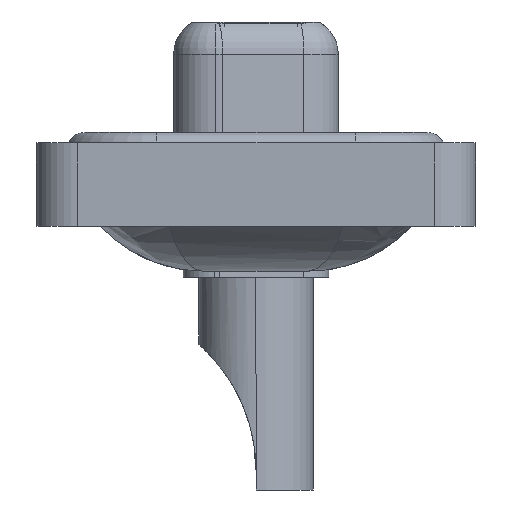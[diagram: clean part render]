
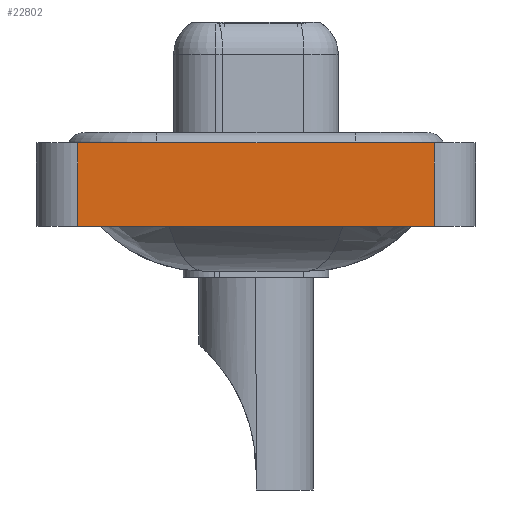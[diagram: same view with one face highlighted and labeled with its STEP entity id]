
A CAD part, left-side view. The second image highlights one B-rep face of the part: STEP entity #22802.
In plain terms, the highlighted planar face has unit normal (-1, 0, 0).
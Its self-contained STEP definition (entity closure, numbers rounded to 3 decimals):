
#503 = LINE ( 'NONE', #8455, #5106 ) ;
#983 = EDGE_CURVE ( 'NONE', #21181, #12863, #14536, .T. ) ;
#1164 = CARTESIAN_POINT ( 'NONE',  ( -7.35, 8.55, -3.6 ) ) ;
#1801 = EDGE_LOOP ( 'NONE', ( #6917, #3983, #19394, #10725 ) ) ;
#2086 = LINE ( 'NONE', #11901, #5328 ) ;
#2424 = VECTOR ( 'NONE', #16769, 1000. ) ;
#3639 = AXIS2_PLACEMENT_3D ( 'NONE', #20539, #20786, #24536 ) ;
#3983 = ORIENTED_EDGE ( 'NONE', *, *, #7214, .F. ) ;
#5106 = VECTOR ( 'NONE', #10077, 1000. ) ;
#5328 = VECTOR ( 'NONE', #9926, 1000. ) ;
#5369 = FACE_OUTER_BOUND ( 'NONE', #1801, .T. ) ;
#6917 = ORIENTED_EDGE ( 'NONE', *, *, #24119, .T. ) ;
#7214 = EDGE_CURVE ( 'NONE', #12863, #23001, #503, .T. ) ;
#8455 = CARTESIAN_POINT ( 'NONE',  ( -7.35, -8.55, 0.4 ) ) ;
#9463 = VERTEX_POINT ( 'NONE', #22011 ) ;
#9675 = DIRECTION ( 'NONE',  ( 0., 0., 1. ) ) ;
#9926 = DIRECTION ( 'NONE',  ( 0., -1., 0. ) ) ;
#10077 = DIRECTION ( 'NONE',  ( 0., -1., 0. ) ) ;
#10725 = ORIENTED_EDGE ( 'NONE', *, *, #20504, .T. ) ;
#11655 = CARTESIAN_POINT ( 'NONE',  ( -7.35, -8.55, -3.6 ) ) ;
#11901 = CARTESIAN_POINT ( 'NONE',  ( -7.35, -8.55, -3.6 ) ) ;
#12857 = VECTOR ( 'NONE', #9675, 1000. ) ;
#12863 = VERTEX_POINT ( 'NONE', #21901 ) ;
#14536 = LINE ( 'NONE', #22486, #2424 ) ;
#16769 = DIRECTION ( 'NONE',  ( 0., 0., 1. ) ) ;
#16937 = PLANE ( 'NONE',  #3639 ) ;
#18297 = CARTESIAN_POINT ( 'NONE',  ( -7.35, -8.55, 0.4 ) ) ;
#19111 = LINE ( 'NONE', #11655, #12857 ) ;
#19394 = ORIENTED_EDGE ( 'NONE', *, *, #983, .F. ) ;
#20504 = EDGE_CURVE ( 'NONE', #21181, #9463, #2086, .T. ) ;
#20539 = CARTESIAN_POINT ( 'NONE',  ( -7.35, -8.55, -3.6 ) ) ;
#20786 = DIRECTION ( 'NONE',  ( -1., 0., 0. ) ) ;
#21181 = VERTEX_POINT ( 'NONE', #1164 ) ;
#21901 = CARTESIAN_POINT ( 'NONE',  ( -7.35, 8.55, 0.4 ) ) ;
#22011 = CARTESIAN_POINT ( 'NONE',  ( -7.35, -8.55, -3.6 ) ) ;
#22486 = CARTESIAN_POINT ( 'NONE',  ( -7.35, 8.55, -3.6 ) ) ;
#22802 = ADVANCED_FACE ( 'NONE', ( #5369 ), #16937, .T. ) ;
#23001 = VERTEX_POINT ( 'NONE', #18297 ) ;
#24119 = EDGE_CURVE ( 'NONE', #9463, #23001, #19111, .T. ) ;
#24536 = DIRECTION ( 'NONE',  ( 0., 0., 1. ) ) ;
